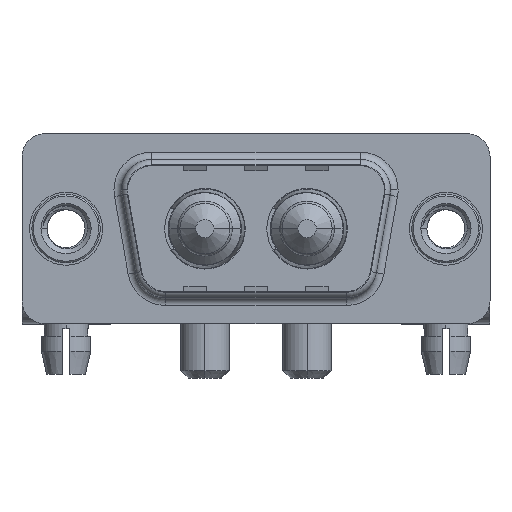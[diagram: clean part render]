
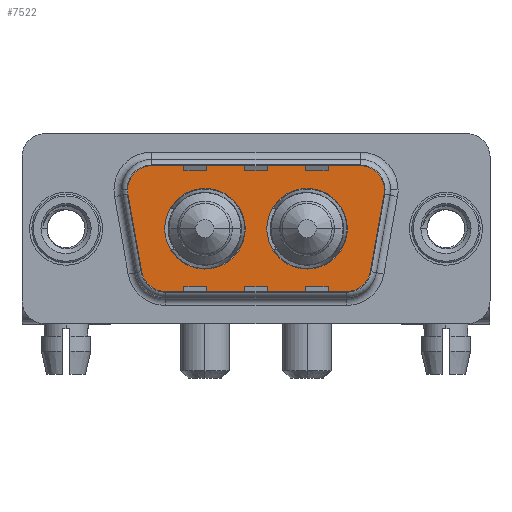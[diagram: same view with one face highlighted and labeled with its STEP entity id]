
A CAD part, top view. The second image highlights one B-rep face of the part: STEP entity #7522.
In plain terms, the highlighted planar face has unit normal (0, 0, 1).
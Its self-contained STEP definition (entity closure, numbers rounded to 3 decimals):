
#23 = CIRCLE ( 'NONE', #10923, 2.65 ) ;
#127 = VERTEX_POINT ( 'NONE', #7744 ) ;
#297 = AXIS2_PLACEMENT_3D ( 'NONE', #14159, #11706, #900 ) ;
#381 = EDGE_CURVE ( 'NONE', #11600, #127, #12768, .T. ) ;
#649 = DIRECTION ( 'NONE',  ( 0.174, 0.985, 0. ) ) ;
#756 = DIRECTION ( 'NONE',  ( 1., 0., 0. ) ) ;
#794 = VERTEX_POINT ( 'NONE', #4964 ) ;
#795 = DIRECTION ( 'NONE',  ( 0., 0., 1. ) ) ;
#809 = CARTESIAN_POINT ( 'NONE',  ( 3.466, 2.553, 0. ) ) ;
#832 = CARTESIAN_POINT ( 'NONE',  ( 15.86, 0., 0. ) ) ;
#888 = DIRECTION ( 'NONE',  ( 1., 0., 0. ) ) ;
#900 = DIRECTION ( 'NONE',  ( -1., 0., 0. ) ) ;
#972 = EDGE_CURVE ( 'NONE', #5030, #13434, #11573, .T. ) ;
#1059 = CIRCLE ( 'NONE', #5889, 2. ) ;
#1232 = VECTOR ( 'NONE', #10373, 1000. ) ;
#1290 = EDGE_CURVE ( 'NONE', #13434, #5030, #15465, .T. ) ;
#1786 = CARTESIAN_POINT ( 'NONE',  ( 15.86, 0., 0. ) ) ;
#1904 = CARTESIAN_POINT ( 'NONE',  ( 5.436, 2.9, 0. ) ) ;
#2079 = DIRECTION ( 'NONE',  ( 0., 0., 1. ) ) ;
#2103 = CIRCLE ( 'NONE', #3626, 2. ) ;
#2154 = LINE ( 'NONE', #809, #7840 ) ;
#2438 = DIRECTION ( 'NONE',  ( -1., 0., 0. ) ) ;
#2837 = EDGE_LOOP ( 'NONE', ( #5374, #11978 ) ) ;
#2844 = EDGE_CURVE ( 'NONE', #794, #10792, #2944, .T. ) ;
#2944 = LINE ( 'NONE', #10403, #10744 ) ;
#2989 = CARTESIAN_POINT ( 'NONE',  ( 3.466, 2.553, 0. ) ) ;
#3132 = DIRECTION ( 'NONE',  ( 0., 0., 1. ) ) ;
#3275 = CARTESIAN_POINT ( 'NONE',  ( 21.534, 2.553, 0. ) ) ;
#3284 = AXIS2_PLACEMENT_3D ( 'NONE', #8112, #2079, #888 ) ;
#3582 = VERTEX_POINT ( 'NONE', #8542 ) ;
#3626 = AXIS2_PLACEMENT_3D ( 'NONE', #1904, #5320, #4450 ) ;
#3630 = EDGE_CURVE ( 'NONE', #13210, #3582, #6727, .T. ) ;
#3673 = ORIENTED_EDGE ( 'NONE', *, *, #10732, .F. ) ;
#4354 = EDGE_LOOP ( 'NONE', ( #7688, #14859, #9216, #7526, #15591, #5961, #12364, #4765, #8596 ) ) ;
#4450 = DIRECTION ( 'NONE',  ( 1., 0., 0. ) ) ;
#4483 = EDGE_CURVE ( 'NONE', #10792, #15051, #13496, .T. ) ;
#4569 = EDGE_CURVE ( 'NONE', #10100, #794, #1059, .T. ) ;
#4765 = ORIENTED_EDGE ( 'NONE', *, *, #3630, .T. ) ;
#4964 = CARTESIAN_POINT ( 'NONE',  ( 20.511, -3.247, 0. ) ) ;
#5030 = VERTEX_POINT ( 'NONE', #15701 ) ;
#5066 = AXIS2_PLACEMENT_3D ( 'NONE', #832, #14325, #756 ) ;
#5320 = DIRECTION ( 'NONE',  ( 0., 0., 1. ) ) ;
#5351 = VERTEX_POINT ( 'NONE', #2989 ) ;
#5374 = ORIENTED_EDGE ( 'NONE', *, *, #972, .F. ) ;
#5731 = DIRECTION ( 'NONE',  ( 0., 0., 1. ) ) ;
#5889 = AXIS2_PLACEMENT_3D ( 'NONE', #14008, #3132, #6793 ) ;
#5961 = ORIENTED_EDGE ( 'NONE', *, *, #14772, .T. ) ;
#6148 = CARTESIAN_POINT ( 'NONE',  ( 6.459, -4.9, 0. ) ) ;
#6669 = CARTESIAN_POINT ( 'NONE',  ( 18.541, -2.9, 0. ) ) ;
#6727 = CIRCLE ( 'NONE', #14314, 2. ) ;
#6793 = DIRECTION ( 'NONE',  ( 1., 0., 0. ) ) ;
#6954 = VERTEX_POINT ( 'NONE', #9227 ) ;
#6968 = CARTESIAN_POINT ( 'NONE',  ( 5.436, 4.9, 0. ) ) ;
#6981 = FACE_OUTER_BOUND ( 'NONE', #4354, .T. ) ;
#7522 = ADVANCED_FACE ( 'NONE', ( #15239, #13009, #6981 ), #12781, .T. ) ;
#7526 = ORIENTED_EDGE ( 'NONE', *, *, #12703, .T. ) ;
#7530 = CARTESIAN_POINT ( 'NONE',  ( 6.49, 0., 0. ) ) ;
#7549 = AXIS2_PLACEMENT_3D ( 'NONE', #6669, #11507, #10304 ) ;
#7684 = ORIENTED_EDGE ( 'NONE', *, *, #12763, .F. ) ;
#7688 = ORIENTED_EDGE ( 'NONE', *, *, #4569, .T. ) ;
#7744 = CARTESIAN_POINT ( 'NONE',  ( 5.436, 4.9, 0. ) ) ;
#7840 = VECTOR ( 'NONE', #11694, 1000. ) ;
#7922 = CARTESIAN_POINT ( 'NONE',  ( 19.564, 4.9, 0. ) ) ;
#8112 = CARTESIAN_POINT ( 'NONE',  ( 9.14, 0., 0. ) ) ;
#8542 = CARTESIAN_POINT ( 'NONE',  ( 6.459, -4.9, 0. ) ) ;
#8596 = ORIENTED_EDGE ( 'NONE', *, *, #13975, .T. ) ;
#8616 = CARTESIAN_POINT ( 'NONE',  ( 6.459, -2.9, 0. ) ) ;
#8685 = CARTESIAN_POINT ( 'NONE',  ( 13.21, 0., 0. ) ) ;
#9144 = VERTEX_POINT ( 'NONE', #7530 ) ;
#9216 = ORIENTED_EDGE ( 'NONE', *, *, #4483, .T. ) ;
#9227 = CARTESIAN_POINT ( 'NONE',  ( 11.79, 0., 0. ) ) ;
#9431 = EDGE_LOOP ( 'NONE', ( #7684, #3673 ) ) ;
#9437 = DIRECTION ( 'NONE',  ( -1., 0., 0. ) ) ;
#10032 = AXIS2_PLACEMENT_3D ( 'NONE', #1786, #12507, #11473 ) ;
#10100 = VERTEX_POINT ( 'NONE', #13509 ) ;
#10304 = DIRECTION ( 'NONE',  ( 1., 0., 0. ) ) ;
#10373 = DIRECTION ( 'NONE',  ( -1., 0., 0. ) ) ;
#10403 = CARTESIAN_POINT ( 'NONE',  ( 21.534, 2.553, 0. ) ) ;
#10558 = DIRECTION ( 'NONE',  ( 1., 0., 0. ) ) ;
#10633 = EDGE_CURVE ( 'NONE', #5351, #13210, #2154, .T. ) ;
#10732 = EDGE_CURVE ( 'NONE', #9144, #6954, #12921, .T. ) ;
#10744 = VECTOR ( 'NONE', #649, 1000. ) ;
#10792 = VERTEX_POINT ( 'NONE', #3275 ) ;
#10923 = AXIS2_PLACEMENT_3D ( 'NONE', #12944, #5731, #10558 ) ;
#11218 = LINE ( 'NONE', #6148, #12469 ) ;
#11473 = DIRECTION ( 'NONE',  ( 1., 0., 0. ) ) ;
#11507 = DIRECTION ( 'NONE',  ( 0., 0., 1. ) ) ;
#11573 = CIRCLE ( 'NONE', #10032, 2.65 ) ;
#11600 = VERTEX_POINT ( 'NONE', #7922 ) ;
#11694 = DIRECTION ( 'NONE',  ( 0.174, -0.985, 0. ) ) ;
#11706 = DIRECTION ( 'NONE',  ( 0., 0., 1. ) ) ;
#11978 = ORIENTED_EDGE ( 'NONE', *, *, #1290, .F. ) ;
#12125 = DIRECTION ( 'NONE',  ( 0., 0., 1. ) ) ;
#12364 = ORIENTED_EDGE ( 'NONE', *, *, #10633, .T. ) ;
#12469 = VECTOR ( 'NONE', #14712, 1000. ) ;
#12507 = DIRECTION ( 'NONE',  ( 0., 0., 1. ) ) ;
#12703 = EDGE_CURVE ( 'NONE', #15051, #11600, #14227, .T. ) ;
#12713 = CARTESIAN_POINT ( 'NONE',  ( 19.564, 2.9, 0. ) ) ;
#12763 = EDGE_CURVE ( 'NONE', #6954, #9144, #23, .T. ) ;
#12768 = LINE ( 'NONE', #6968, #1232 ) ;
#12781 = PLANE ( 'NONE',  #7549 ) ;
#12921 = CIRCLE ( 'NONE', #3284, 2.65 ) ;
#12944 = CARTESIAN_POINT ( 'NONE',  ( 9.14, 0., 0. ) ) ;
#13009 = FACE_BOUND ( 'NONE', #9431, .T. ) ;
#13210 = VERTEX_POINT ( 'NONE', #15315 ) ;
#13434 = VERTEX_POINT ( 'NONE', #8685 ) ;
#13496 = CIRCLE ( 'NONE', #297, 2. ) ;
#13509 = CARTESIAN_POINT ( 'NONE',  ( 18.541, -4.9, 0. ) ) ;
#13975 = EDGE_CURVE ( 'NONE', #3582, #10100, #11218, .T. ) ;
#14008 = CARTESIAN_POINT ( 'NONE',  ( 18.541, -2.9, 0. ) ) ;
#14159 = CARTESIAN_POINT ( 'NONE',  ( 19.564, 2.9, 0. ) ) ;
#14227 = CIRCLE ( 'NONE', #14718, 2. ) ;
#14314 = AXIS2_PLACEMENT_3D ( 'NONE', #8616, #12125, #2438 ) ;
#14325 = DIRECTION ( 'NONE',  ( 0., 0., 1. ) ) ;
#14712 = DIRECTION ( 'NONE',  ( 1., 0., 0. ) ) ;
#14718 = AXIS2_PLACEMENT_3D ( 'NONE', #12713, #795, #9437 ) ;
#14772 = EDGE_CURVE ( 'NONE', #127, #5351, #2103, .T. ) ;
#14859 = ORIENTED_EDGE ( 'NONE', *, *, #2844, .T. ) ;
#14901 = CARTESIAN_POINT ( 'NONE',  ( 21.564, 2.9, 0. ) ) ;
#15051 = VERTEX_POINT ( 'NONE', #14901 ) ;
#15239 = FACE_BOUND ( 'NONE', #2837, .T. ) ;
#15315 = CARTESIAN_POINT ( 'NONE',  ( 4.489, -3.247, 0. ) ) ;
#15465 = CIRCLE ( 'NONE', #5066, 2.65 ) ;
#15591 = ORIENTED_EDGE ( 'NONE', *, *, #381, .T. ) ;
#15701 = CARTESIAN_POINT ( 'NONE',  ( 18.51, 0., 0. ) ) ;
